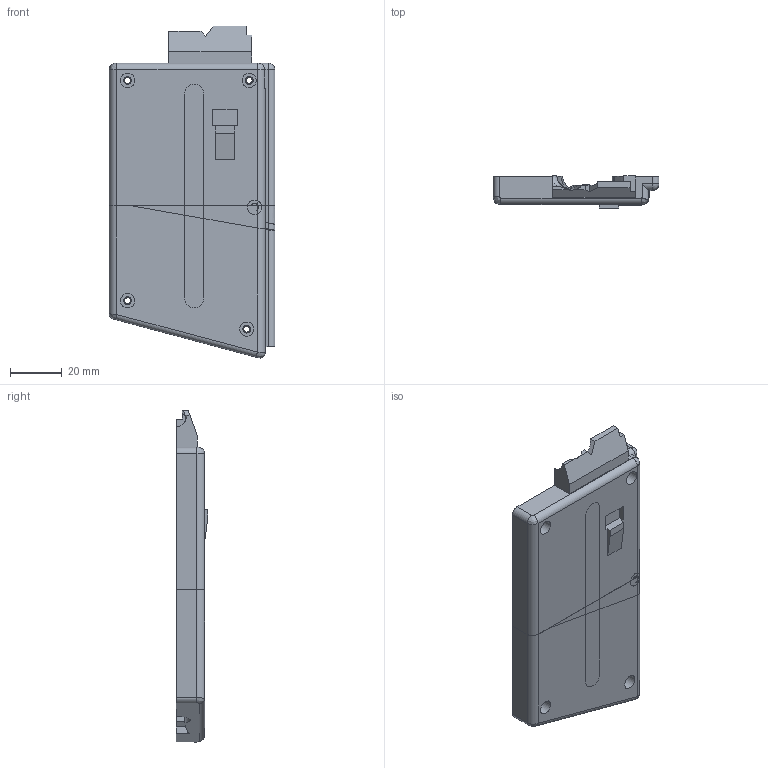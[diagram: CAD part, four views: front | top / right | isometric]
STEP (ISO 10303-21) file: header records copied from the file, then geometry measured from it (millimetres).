
FILE_DESCRIPTION(/* description */ (''),/* implementation_level */ '2;1');
FILE_NAME(/* name */ 'Left Body.step',/* time_stamp */ '2020-05-29T15:49:40-04:00',/* author */ (''),/* organization */ (''),/* preprocessor_version */ 'ST-DEVELOPER v18.1',/* originating_system */ 'Autodesk Translation Framework v9.3.0.1241',/* authorisation */ '');
FILE_SCHEMA (('AUTOMOTIVE_DESIGN { 1 0 10303 214 3 1 1 }'));
Products named in the file (1): Left Body
Bounding box: 64 x 12.32 x 128.15 mm (x, y, z)
Volume: 63160.6 mm3; surface area: 25973.3 mm2
Topology: 10 solids, 10 shells, 515 faces, 1443 edges, 953 vertices
Faces by surface type: cylinder 241, bspline 135, plane 119, cone 19, sphere 1
Full cylindrical faces by diameter (mm): 2.35 x48, 3 x52, 5.5 x4
Entity records: 105835 total; most frequent: CARTESIAN_POINT 94396, ORIENTED_EDGE 2886, DIRECTION 1610, EDGE_CURVE 1443, VERTEX_POINT 953, B_SPLINE_CURVE_WITH_KNOTS 701, LINE 562, VECTOR 562
